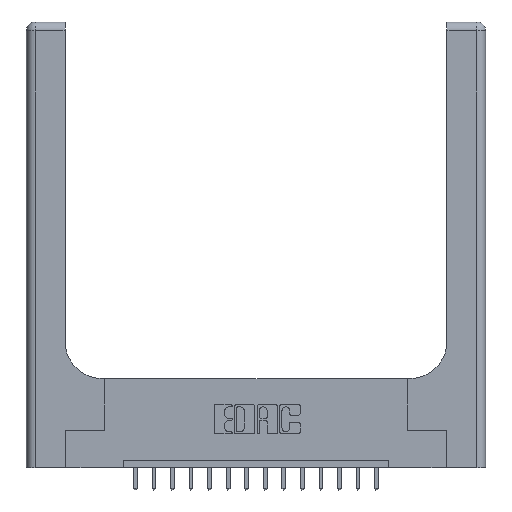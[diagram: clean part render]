
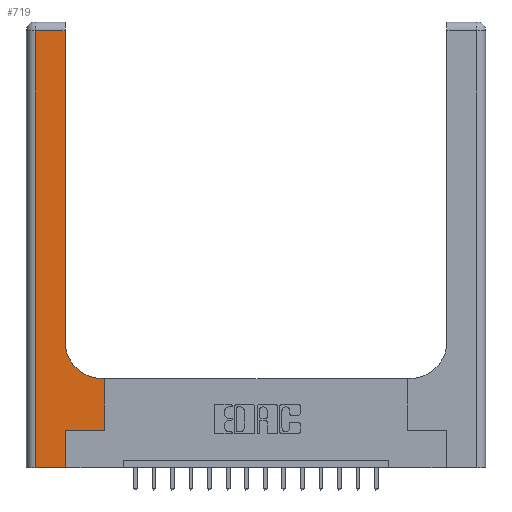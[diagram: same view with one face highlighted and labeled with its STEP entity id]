
A CAD part, top view. The second image highlights one B-rep face of the part: STEP entity #719.
In plain terms, the highlighted planar face has unit normal (0, 0, 1).
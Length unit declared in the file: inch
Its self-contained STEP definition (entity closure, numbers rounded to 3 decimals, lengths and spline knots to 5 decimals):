
#38 = CARTESIAN_POINT ( 'NONE',  ( 0.265, 0.25, 0.37 ) ) ;
#52 = CARTESIAN_POINT ( 'NONE',  ( 0.06, 0., 0.37 ) ) ;
#219 = LINE ( 'NONE', #2865, #635 ) ;
#425 = CARTESIAN_POINT ( 'NONE',  ( 0.528, 0.6, 0.37 ) ) ;
#437 = ORIENTED_EDGE ( 'NONE', *, *, #10468, .T. ) ;
#635 = VECTOR ( 'NONE', #7335, 39.37008 ) ;
#719 = ADVANCED_FACE ( 'NONE', ( #1584 ), #9742, .F. ) ;
#765 = ORIENTED_EDGE ( 'NONE', *, *, #12976, .T. ) ;
#856 = CIRCLE ( 'NONE', #8167, 0.25 ) ;
#1174 = CARTESIAN_POINT ( 'NONE',  ( 0.265, 0.25, 0.37 ) ) ;
#1245 = CARTESIAN_POINT ( 'NONE',  ( 0.06, 3., 0.37 ) ) ;
#1584 = FACE_OUTER_BOUND ( 'NONE', #1746, .T. ) ;
#1645 = VERTEX_POINT ( 'NONE', #7901 ) ;
#1671 = DIRECTION ( 'NONE',  ( -1., 0., 0. ) ) ;
#1746 = EDGE_LOOP ( 'NONE', ( #15598, #5817, #6444, #765, #10898, #4664, #437, #4291, #14680 ) ) ;
#1814 = EDGE_CURVE ( 'NONE', #5661, #13003, #219, .T. ) ;
#1883 = DIRECTION ( 'NONE',  ( 0., 1., 0. ) ) ;
#2363 = LINE ( 'NONE', #1174, #5560 ) ;
#2570 = VERTEX_POINT ( 'NONE', #9507 ) ;
#2572 = VERTEX_POINT ( 'NONE', #13722 ) ;
#2682 = AXIS2_PLACEMENT_3D ( 'NONE', #11280, #15604, #1671 ) ;
#2728 = EDGE_CURVE ( 'NONE', #2572, #4528, #4629, .T. ) ;
#2835 = EDGE_CURVE ( 'NONE', #13003, #15504, #12335, .T. ) ;
#2865 = CARTESIAN_POINT ( 'NONE',  ( 0., 2.94, 0.37 ) ) ;
#3074 = LINE ( 'NONE', #8652, #6530 ) ;
#3076 = DIRECTION ( 'NONE',  ( 0., 1., 0. ) ) ;
#3431 = CARTESIAN_POINT ( 'NONE',  ( 0.06, 2.94, 0.37 ) ) ;
#3451 = DIRECTION ( 'NONE',  ( 0., 0., -1. ) ) ;
#3936 = LINE ( 'NONE', #5930, #9627 ) ;
#4291 = ORIENTED_EDGE ( 'NONE', *, *, #6776, .T. ) ;
#4387 = DIRECTION ( 'NONE',  ( 0., 1., 0. ) ) ;
#4528 = VERTEX_POINT ( 'NONE', #38 ) ;
#4629 = LINE ( 'NONE', #15637, #15577 ) ;
#4664 = ORIENTED_EDGE ( 'NONE', *, *, #7474, .T. ) ;
#5560 = VECTOR ( 'NONE', #13542, 39.37008 ) ;
#5584 = VERTEX_POINT ( 'NONE', #13283 ) ;
#5661 = VERTEX_POINT ( 'NONE', #16025 ) ;
#5817 = ORIENTED_EDGE ( 'NONE', *, *, #1814, .T. ) ;
#5930 = CARTESIAN_POINT ( 'NONE',  ( 0.26, 3., 0.37 ) ) ;
#6444 = ORIENTED_EDGE ( 'NONE', *, *, #2835, .T. ) ;
#6470 = DIRECTION ( 'NONE',  ( 1., 0., 0. ) ) ;
#6530 = VECTOR ( 'NONE', #1883, 39.37008 ) ;
#6776 = EDGE_CURVE ( 'NONE', #10588, #2570, #6983, .T. ) ;
#6820 = DIRECTION ( 'NONE',  ( 0., -1., 0. ) ) ;
#6983 = LINE ( 'NONE', #13788, #15466 ) ;
#7335 = DIRECTION ( 'NONE',  ( -1., 0., 0. ) ) ;
#7436 = LINE ( 'NONE', #17084, #11289 ) ;
#7474 = EDGE_CURVE ( 'NONE', #4528, #5584, #2363, .T. ) ;
#7901 = CARTESIAN_POINT ( 'NONE',  ( 0.26, 0.85, 0.37 ) ) ;
#7955 = VECTOR ( 'NONE', #6820, 39.37008 ) ;
#8167 = AXIS2_PLACEMENT_3D ( 'NONE', #15995, #3451, #6470 ) ;
#8652 = CARTESIAN_POINT ( 'NONE',  ( 0.528, 0.25, 0.37 ) ) ;
#9507 = CARTESIAN_POINT ( 'NONE',  ( 0.51, 0.6, 0.37 ) ) ;
#9627 = VECTOR ( 'NONE', #4387, 39.37008 ) ;
#9742 = PLANE ( 'NONE',  #2682 ) ;
#9830 = DIRECTION ( 'NONE',  ( -1., 0., 0. ) ) ;
#10468 = EDGE_CURVE ( 'NONE', #5584, #10588, #3074, .T. ) ;
#10588 = VERTEX_POINT ( 'NONE', #425 ) ;
#10898 = ORIENTED_EDGE ( 'NONE', *, *, #2728, .T. ) ;
#11280 = CARTESIAN_POINT ( 'NONE',  ( 0., 3., 0.37 ) ) ;
#11289 = VECTOR ( 'NONE', #12870, 39.37008 ) ;
#12335 = LINE ( 'NONE', #1245, #7955 ) ;
#12870 = DIRECTION ( 'NONE',  ( 1., 0., 0. ) ) ;
#12976 = EDGE_CURVE ( 'NONE', #15504, #2572, #7436, .T. ) ;
#13003 = VERTEX_POINT ( 'NONE', #3431 ) ;
#13283 = CARTESIAN_POINT ( 'NONE',  ( 0.528, 0.25, 0.37 ) ) ;
#13542 = DIRECTION ( 'NONE',  ( 1., 0., 0. ) ) ;
#13722 = CARTESIAN_POINT ( 'NONE',  ( 0.265, 0., 0.37 ) ) ;
#13788 = CARTESIAN_POINT ( 'NONE',  ( 0.26, 0.6, 0.37 ) ) ;
#14680 = ORIENTED_EDGE ( 'NONE', *, *, #16184, .T. ) ;
#15466 = VECTOR ( 'NONE', #9830, 39.37008 ) ;
#15504 = VERTEX_POINT ( 'NONE', #52 ) ;
#15577 = VECTOR ( 'NONE', #3076, 39.37008 ) ;
#15598 = ORIENTED_EDGE ( 'NONE', *, *, #17692, .T. ) ;
#15604 = DIRECTION ( 'NONE',  ( 0., 0., -1. ) ) ;
#15637 = CARTESIAN_POINT ( 'NONE',  ( 0.265, 0., 0.37 ) ) ;
#15995 = CARTESIAN_POINT ( 'NONE',  ( 0.51, 0.85, 0.37 ) ) ;
#16025 = CARTESIAN_POINT ( 'NONE',  ( 0.26, 2.94, 0.37 ) ) ;
#16184 = EDGE_CURVE ( 'NONE', #2570, #1645, #856, .T. ) ;
#17084 = CARTESIAN_POINT ( 'NONE',  ( 0., 0., 0.37 ) ) ;
#17692 = EDGE_CURVE ( 'NONE', #1645, #5661, #3936, .T. ) ;
